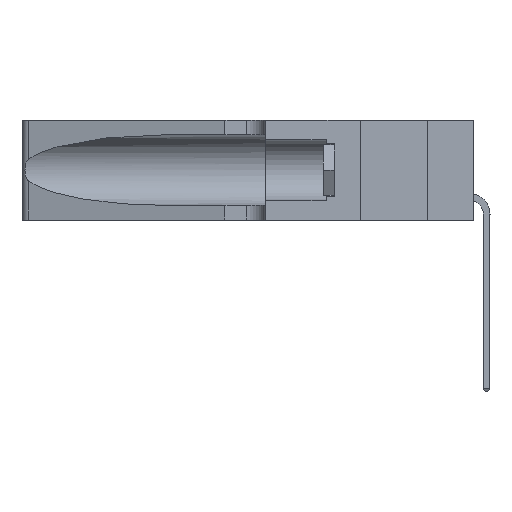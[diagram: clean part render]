
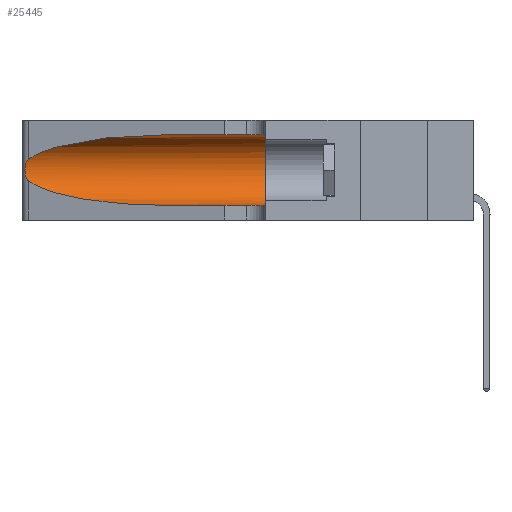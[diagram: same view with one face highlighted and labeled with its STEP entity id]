
A CAD part, left-side view. The second image highlights one B-rep face of the part: STEP entity #25445.
In plain terms, the highlighted cylindrical face has radius 3.308 mm (diameter 6.617 mm), a partial arc.
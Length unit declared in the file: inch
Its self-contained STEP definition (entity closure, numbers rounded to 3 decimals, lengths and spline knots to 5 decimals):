
#959 = AXIS2_PLACEMENT_3D ( 'NONE', #9720, #42718, #35060 ) ;
#1092 = VERTEX_POINT ( 'NONE', #46478 ) ;
#1141 = EDGE_CURVE ( 'NONE', #40216, #1092, #22077, .T. ) ;
#1954 = CARTESIAN_POINT ( 'NONE',  ( 0.1305, 1.61858, 0.185 ) ) ;
#1955 = EDGE_LOOP ( 'NONE', ( #35124, #32980, #36855, #8513, #10451, #25921 ) ) ;
#2874 = VECTOR ( 'NONE', #23537, 39.37008 ) ;
#3559 = CARTESIAN_POINT ( 'NONE',  ( 0.25639, 1.23186, 0.15144 ) ) ;
#5273 = CARTESIAN_POINT ( 'NONE',  ( 0.1305, 0.72297, 0.31525 ) ) ;
#5469 = VERTEX_POINT ( 'NONE', #38793 ) ;
#7205 = CARTESIAN_POINT ( 'NONE',  ( 0.26075, 1.23896, 0.178 ) ) ;
#8286 = EDGE_CURVE ( 'NONE', #15666, #40216, #29616, .T. ) ;
#8513 = ORIENTED_EDGE ( 'NONE', *, *, #16014, .T. ) ;
#9720 = CARTESIAN_POINT ( 'NONE',  ( 0.1305, 0.35, 0.185 ) ) ;
#10294 = LINE ( 'NONE', #35075, #2874 ) ;
#10451 = ORIENTED_EDGE ( 'NONE', *, *, #35623, .F. ) ;
#10682 = CARTESIAN_POINT ( 'NONE',  ( 0.26075, 1.23896, 0.19203 ) ) ;
#10795 = CARTESIAN_POINT ( 'NONE',  ( 0.2373, 1.15595, 0.08982 ) ) ;
#10877 = CARTESIAN_POINT ( 'NONE',  ( 0.25789, 1.23486, 0.15765 ) ) ;
#11358 = CARTESIAN_POINT ( 'NONE',  ( 0.18966, 0.96281, 0.05475 ) ) ;
#11752 = VERTEX_POINT ( 'NONE', #29775 ) ;
#14246 = CARTESIAN_POINT ( 'NONE',  ( 0.25639, 1.23184, 0.21858 ) ) ;
#14342 =( BOUNDED_CURVE ( )  B_SPLINE_CURVE ( 3, ( #18687, #10795, #11358, #40361 ),
 .UNSPECIFIED., .F., .F. ) 
 B_SPLINE_CURVE_WITH_KNOTS ( ( 4, 4 ),
 ( 3.44316, 4.71239 ),
 .UNSPECIFIED. ) 
 CURVE ( )  GEOMETRIC_REPRESENTATION_ITEM ( )  RATIONAL_B_SPLINE_CURVE ( ( 1., 0.87, 0.87, 1. ) ) 
 REPRESENTATION_ITEM ( '' )  );
#15285 = VECTOR ( 'NONE', #45430, 39.37008 ) ;
#15666 = VERTEX_POINT ( 'NONE', #38927 ) ;
#16014 = EDGE_CURVE ( 'NONE', #30353, #5469, #10294, .T. ) ;
#16264 = CARTESIAN_POINT ( 'NONE',  ( 0.2373, 1.15595, 0.28018 ) ) ;
#17218 = EDGE_CURVE ( 'NONE', #15666, #11752, #46488, .T. ) ;
#17592 = FACE_OUTER_BOUND ( 'NONE', #1955, .T. ) ;
#18687 = CARTESIAN_POINT ( 'NONE',  ( 0.25487, 1.22718, 0.14631 ) ) ;
#19206 = CYLINDRICAL_SURFACE ( 'NONE', #30828, 0.13025 ) ;
#19874 = CARTESIAN_POINT ( 'NONE',  ( 0.25487, 1.22718, 0.22369 ) ) ;
#20124 = CARTESIAN_POINT ( 'NONE',  ( 0.1305, 1.61858, 0.31525 ) ) ;
#21510 = CARTESIAN_POINT ( 'NONE',  ( 0.25854, 1.2359, 0.20912 ) ) ;
#21793 = CARTESIAN_POINT ( 'NONE',  ( 0.25787, 1.23484, 0.2124 ) ) ;
#22077 = B_SPLINE_CURVE_WITH_KNOTS ( 'NONE', 3,
 ( #28434, #39387, #14246, #21793, #21510, #25126, #10682, #7205, #29034, #36076, #10877, #3559, #45159, #23986 ),
 .UNSPECIFIED., .F., .F.,
 ( 4, 2, 2, 2, 2, 2, 4 ),
 ( 0., 0.00027, 0.00053, 0.00107, 0.0016, 0.00187, 0.00214 ),
 .UNSPECIFIED. ) ;
#23537 = DIRECTION ( 'NONE',  ( 0., -1., 0. ) ) ;
#23986 = CARTESIAN_POINT ( 'NONE',  ( 0.25487, 1.22718, 0.14631 ) ) ;
#25126 = CARTESIAN_POINT ( 'NONE',  ( 0.26018, 1.23835, 0.19895 ) ) ;
#25445 = ADVANCED_FACE ( 'NONE', ( #17592 ), #19206, .F. ) ;
#25477 = CARTESIAN_POINT ( 'NONE',  ( 0.25487, 1.22718, 0.22369 ) ) ;
#25921 = ORIENTED_EDGE ( 'NONE', *, *, #17218, .F. ) ;
#28434 = CARTESIAN_POINT ( 'NONE',  ( 0.25487, 1.22718, 0.22369 ) ) ;
#29034 = CARTESIAN_POINT ( 'NONE',  ( 0.26017, 1.23833, 0.17102 ) ) ;
#29616 =( BOUNDED_CURVE ( )  B_SPLINE_CURVE ( 3, ( #5273, #34256, #16264, #19874 ),
 .UNSPECIFIED., .F., .F. ) 
 B_SPLINE_CURVE_WITH_KNOTS ( ( 4, 4 ),
 ( 1.5708, 2.84003 ),
 .UNSPECIFIED. ) 
 CURVE ( )  GEOMETRIC_REPRESENTATION_ITEM ( )  RATIONAL_B_SPLINE_CURVE ( ( 1., 0.87, 0.87, 1. ) ) 
 REPRESENTATION_ITEM ( '' )  );
#29775 = CARTESIAN_POINT ( 'NONE',  ( 0.1305, 0.35, 0.31525 ) ) ;
#30353 = VERTEX_POINT ( 'NONE', #37966 ) ;
#30828 = AXIS2_PLACEMENT_3D ( 'NONE', #1954, #37215, #44306 ) ;
#32980 = ORIENTED_EDGE ( 'NONE', *, *, #1141, .T. ) ;
#34256 = CARTESIAN_POINT ( 'NONE',  ( 0.18966, 0.96281, 0.31525 ) ) ;
#35060 = DIRECTION ( 'NONE',  ( 0., 0., 1. ) ) ;
#35075 = CARTESIAN_POINT ( 'NONE',  ( 0.1305, 1.61858, 0.05475 ) ) ;
#35124 = ORIENTED_EDGE ( 'NONE', *, *, #8286, .T. ) ;
#35623 = EDGE_CURVE ( 'NONE', #11752, #5469, #37812, .T. ) ;
#36076 = CARTESIAN_POINT ( 'NONE',  ( 0.25856, 1.23593, 0.16098 ) ) ;
#36855 = ORIENTED_EDGE ( 'NONE', *, *, #39149, .T. ) ;
#37215 = DIRECTION ( 'NONE',  ( 0., -1., 0. ) ) ;
#37812 = CIRCLE ( 'NONE', #959, 0.13025 ) ;
#37966 = CARTESIAN_POINT ( 'NONE',  ( 0.1305, 0.72297, 0.05475 ) ) ;
#38793 = CARTESIAN_POINT ( 'NONE',  ( 0.1305, 0.35, 0.05475 ) ) ;
#38927 = CARTESIAN_POINT ( 'NONE',  ( 0.1305, 0.72297, 0.31525 ) ) ;
#39149 = EDGE_CURVE ( 'NONE', #1092, #30353, #14342, .T. ) ;
#39387 = CARTESIAN_POINT ( 'NONE',  ( 0.25555, 1.22994, 0.2215 ) ) ;
#40216 = VERTEX_POINT ( 'NONE', #25477 ) ;
#40361 = CARTESIAN_POINT ( 'NONE',  ( 0.1305, 0.72297, 0.05475 ) ) ;
#42718 = DIRECTION ( 'NONE',  ( 0., 1., 0. ) ) ;
#44306 = DIRECTION ( 'NONE',  ( 0., 0., -1. ) ) ;
#45159 = CARTESIAN_POINT ( 'NONE',  ( 0.25555, 1.22993, 0.14849 ) ) ;
#45430 = DIRECTION ( 'NONE',  ( 0., -1., 0. ) ) ;
#46478 = CARTESIAN_POINT ( 'NONE',  ( 0.25487, 1.22718, 0.14631 ) ) ;
#46488 = LINE ( 'NONE', #20124, #15285 ) ;
